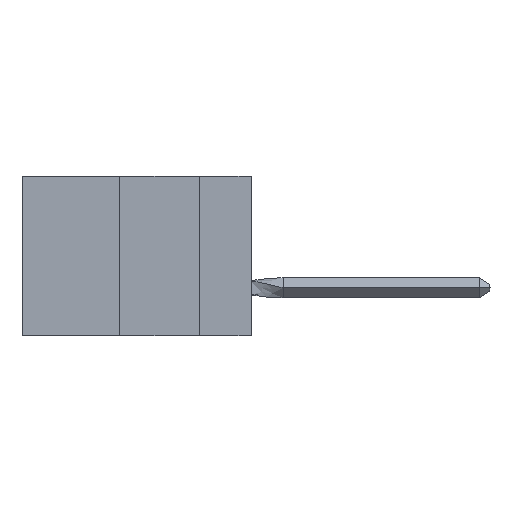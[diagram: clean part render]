
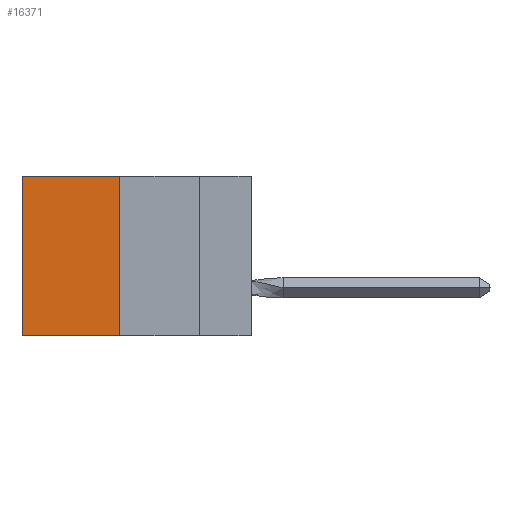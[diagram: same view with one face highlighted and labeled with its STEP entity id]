
A CAD part, left-side view. The second image highlights one B-rep face of the part: STEP entity #16371.
In plain terms, the highlighted planar face has unit normal (-1, 0, 0).
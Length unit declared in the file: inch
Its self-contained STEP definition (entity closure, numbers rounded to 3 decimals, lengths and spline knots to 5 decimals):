
#1179 = DIRECTION ( 'NONE',  ( 0., 0., -1. ) ) ;
#1577 = CARTESIAN_POINT ( 'NONE',  ( 0.305, 0.413, -0.5 ) ) ;
#2745 = CARTESIAN_POINT ( 'NONE',  ( 0.305, 0.413, -0.5 ) ) ;
#3320 = LINE ( 'NONE', #31924, #12814 ) ;
#5175 = LINE ( 'NONE', #2745, #37346 ) ;
#5282 = ORIENTED_EDGE ( 'NONE', *, *, #24457, .F. ) ;
#8979 = ORIENTED_EDGE ( 'NONE', *, *, #26560, .F. ) ;
#9604 = VECTOR ( 'NONE', #14999, 39.37008 ) ;
#12814 = VECTOR ( 'NONE', #37910, 39.37008 ) ;
#12868 = ORIENTED_EDGE ( 'NONE', *, *, #17814, .T. ) ;
#14999 = DIRECTION ( 'NONE',  ( 0., 0., -1. ) ) ;
#15286 = CARTESIAN_POINT ( 'NONE',  ( 0.305, 0.413, 0. ) ) ;
#16371 = ADVANCED_FACE ( 'NONE', ( #26954 ), #22854, .F. ) ;
#17814 = EDGE_CURVE ( 'NONE', #22871, #19849, #24438, .T. ) ;
#18326 = DIRECTION ( 'NONE',  ( 0., 1., 0. ) ) ;
#18733 = CARTESIAN_POINT ( 'NONE',  ( 0.305, 0.413, 0. ) ) ;
#19278 = CARTESIAN_POINT ( 'NONE',  ( 0.305, 0.413, -0.5 ) ) ;
#19849 = VERTEX_POINT ( 'NONE', #32888 ) ;
#20328 = ORIENTED_EDGE ( 'NONE', *, *, #24243, .T. ) ;
#20556 = CARTESIAN_POINT ( 'NONE',  ( 0.305, 0.413, -0.5 ) ) ;
#20709 = EDGE_LOOP ( 'NONE', ( #20328, #5282, #8979, #12868 ) ) ;
#22713 = AXIS2_PLACEMENT_3D ( 'NONE', #19278, #28252, #1179 ) ;
#22854 = PLANE ( 'NONE',  #22713 ) ;
#22871 = VERTEX_POINT ( 'NONE', #18733 ) ;
#24243 = EDGE_CURVE ( 'NONE', #19849, #32607, #3320, .T. ) ;
#24438 = LINE ( 'NONE', #15286, #35340 ) ;
#24457 = EDGE_CURVE ( 'NONE', #36562, #32607, #5175, .T. ) ;
#26560 = EDGE_CURVE ( 'NONE', #22871, #36562, #30797, .T. ) ;
#26954 = FACE_OUTER_BOUND ( 'NONE', #20709, .T. ) ;
#28252 = DIRECTION ( 'NONE',  ( 1., 0., 0. ) ) ;
#30797 = LINE ( 'NONE', #20556, #9604 ) ;
#31924 = CARTESIAN_POINT ( 'NONE',  ( 0.305, 0.72, -0.5 ) ) ;
#32607 = VERTEX_POINT ( 'NONE', #37632 ) ;
#32888 = CARTESIAN_POINT ( 'NONE',  ( 0.305, 0.72, 0. ) ) ;
#33870 = DIRECTION ( 'NONE',  ( 0., 1., 0. ) ) ;
#35340 = VECTOR ( 'NONE', #33870, 39.37008 ) ;
#36562 = VERTEX_POINT ( 'NONE', #1577 ) ;
#37346 = VECTOR ( 'NONE', #18326, 39.37008 ) ;
#37632 = CARTESIAN_POINT ( 'NONE',  ( 0.305, 0.72, -0.5 ) ) ;
#37910 = DIRECTION ( 'NONE',  ( 0., 0., -1. ) ) ;
